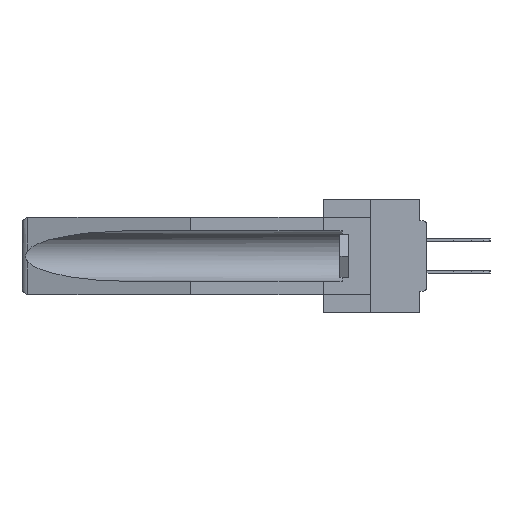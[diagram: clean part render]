
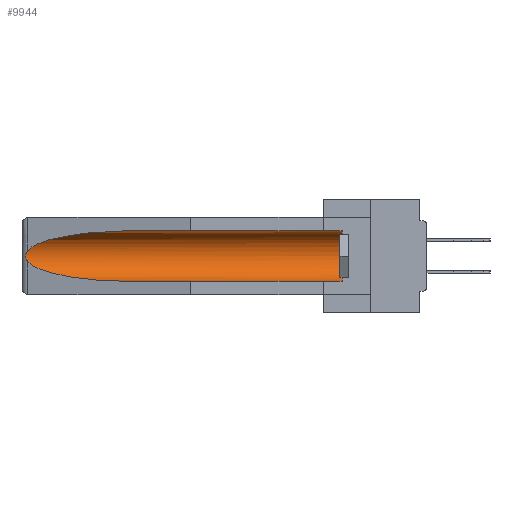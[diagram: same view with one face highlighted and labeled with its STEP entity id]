
A CAD part, left-side view. The second image highlights one B-rep face of the part: STEP entity #9944.
In plain terms, the highlighted cylindrical face has radius 2.857 mm (diameter 5.715 mm), a partial arc.
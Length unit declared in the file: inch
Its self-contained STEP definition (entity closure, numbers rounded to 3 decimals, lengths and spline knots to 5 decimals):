
#399 = CARTESIAN_POINT ( 'NONE',  ( 0.21114, 1.30732, -0.059 ) ) ;
#530 = CARTESIAN_POINT ( 'NONE',  ( 0.155, 1.07973, -0.059 ) ) ;
#977 = DIRECTION ( 'NONE',  ( 0., 1., 0. ) ) ;
#3396 = CARTESIAN_POINT ( 'NONE',  ( 0.25451, 1.48313, -0.09465 ) ) ;
#3493 = CARTESIAN_POINT ( 'NONE',  ( 0.26537, 1.52718, -0.14972 ) ) ;
#3659 = CARTESIAN_POINT ( 'NONE',  ( 0.2673, 1.53269, -0.17917 ) ) ;
#4234 = CARTESIAN_POINT ( 'NONE',  ( 0.155, -0.30754, -0.059 ) ) ;
#4353 = CARTESIAN_POINT ( 'NONE',  ( 0.155, 1.07973, -0.284 ) ) ;
#4997 = VERTEX_POINT ( 'NONE', #4353 ) ;
#5021 = DIRECTION ( 'NONE',  ( 0., -1., 0. ) ) ;
#6024 = CARTESIAN_POINT ( 'NONE',  ( 0.155, 0.126, -0.284 ) ) ;
#6068 = CARTESIAN_POINT ( 'NONE',  ( 0.21114, 1.30732, -0.284 ) ) ;
#7040 = CARTESIAN_POINT ( 'NONE',  ( 0.26654, 1.53092, -0.15636 ) ) ;
#7244 = VERTEX_POINT ( 'NONE', #14159 ) ;
#7848 = CARTESIAN_POINT ( 'NONE',  ( 0.155, 0.126, -0.059 ) ) ;
#7943 = DIRECTION ( 'NONE',  ( 0., 0., 1. ) ) ;
#8507 = AXIS2_PLACEMENT_3D ( 'NONE', #30122, #5021, #26996 ) ;
#8982 = EDGE_CURVE ( 'NONE', #31421, #26354, #31201, .T. ) ;
#9366 = LINE ( 'NONE', #28164, #28283 ) ;
#9666 = ORIENTED_EDGE ( 'NONE', *, *, #23422, .T. ) ;
#9944 = ADVANCED_FACE ( 'NONE', ( #39480 ), #27773, .F. ) ;
#10310 = CARTESIAN_POINT ( 'NONE',  ( 0.2675, 1.53308, -0.17534 ) ) ;
#11092 =( BOUNDED_CURVE ( )  B_SPLINE_CURVE ( 3, ( #27252, #21374, #6068, #27779 ),
 .UNSPECIFIED., .F., .F. ) 
 B_SPLINE_CURVE_WITH_KNOTS ( ( 4, 4 ),
 ( 0.1948, 1.5708 ),
 .UNSPECIFIED. ) 
 CURVE ( )  GEOMETRIC_REPRESENTATION_ITEM ( )  RATIONAL_B_SPLINE_CURVE ( ( 1., 0.848, 0.848, 1. ) ) 
 REPRESENTATION_ITEM ( '' )  );
#14079 = DIRECTION ( 'NONE',  ( 0., 1., 0. ) ) ;
#14159 = CARTESIAN_POINT ( 'NONE',  ( 0.26537, 1.52718, -0.19328 ) ) ;
#14530 = CARTESIAN_POINT ( 'NONE',  ( 0.155, 1.07973, -0.059 ) ) ;
#15015 = EDGE_CURVE ( 'NONE', #18121, #7244, #38730, .T. ) ;
#16290 = CARTESIAN_POINT ( 'NONE',  ( 0.26597, 1.5296, -0.19026 ) ) ;
#16415 = CARTESIAN_POINT ( 'NONE',  ( 0.26537, 1.52718, -0.14972 ) ) ;
#16559 = EDGE_CURVE ( 'NONE', #31421, #4997, #9366, .T. ) ;
#17382 = AXIS2_PLACEMENT_3D ( 'NONE', #26665, #14079, #7943 ) ;
#18121 = VERTEX_POINT ( 'NONE', #3493 ) ;
#18187 = EDGE_LOOP ( 'NONE', ( #9666, #18759, #21582, #34734, #25890, #39552 ) ) ;
#18759 = ORIENTED_EDGE ( 'NONE', *, *, #15015, .T. ) ;
#18803 = DIRECTION ( 'NONE',  ( 0., 1., 0. ) ) ;
#19403 = CARTESIAN_POINT ( 'NONE',  ( 0.26655, 1.53094, -0.18657 ) ) ;
#19683 = VERTEX_POINT ( 'NONE', #14530 ) ;
#21374 = CARTESIAN_POINT ( 'NONE',  ( 0.25451, 1.48313, -0.24835 ) ) ;
#21582 = ORIENTED_EDGE ( 'NONE', *, *, #37620, .T. ) ;
#22199 = CARTESIAN_POINT ( 'NONE',  ( 0.26597, 1.52961, -0.15275 ) ) ;
#23422 = EDGE_CURVE ( 'NONE', #19683, #18121, #24262, .T. ) ;
#24262 =( BOUNDED_CURVE ( )  B_SPLINE_CURVE ( 3, ( #530, #399, #3396, #27813 ),
 .UNSPECIFIED., .F., .F. ) 
 B_SPLINE_CURVE_WITH_KNOTS ( ( 4, 4 ),
 ( 4.71239, 6.08839 ),
 .UNSPECIFIED. ) 
 CURVE ( )  GEOMETRIC_REPRESENTATION_ITEM ( )  RATIONAL_B_SPLINE_CURVE ( ( 1., 0.848, 0.848, 1. ) ) 
 REPRESENTATION_ITEM ( '' )  );
#25419 = VECTOR ( 'NONE', #977, 39.37008 ) ;
#25488 = CARTESIAN_POINT ( 'NONE',  ( 0.2673, 1.5327, -0.16383 ) ) ;
#25885 = CARTESIAN_POINT ( 'NONE',  ( 0.26537, 1.52718, -0.19328 ) ) ;
#25890 = ORIENTED_EDGE ( 'NONE', *, *, #8982, .T. ) ;
#26354 = VERTEX_POINT ( 'NONE', #7848 ) ;
#26665 = CARTESIAN_POINT ( 'NONE',  ( 0.155, -0.30754, -0.1715 ) ) ;
#26996 = DIRECTION ( 'NONE',  ( 0., 0., 1. ) ) ;
#27252 = CARTESIAN_POINT ( 'NONE',  ( 0.26537, 1.52718, -0.19328 ) ) ;
#27773 = CYLINDRICAL_SURFACE ( 'NONE', #17382, 0.1125 ) ;
#27779 = CARTESIAN_POINT ( 'NONE',  ( 0.155, 1.07973, -0.284 ) ) ;
#27813 = CARTESIAN_POINT ( 'NONE',  ( 0.26537, 1.52718, -0.14972 ) ) ;
#28164 = CARTESIAN_POINT ( 'NONE',  ( 0.155, -0.30754, -0.284 ) ) ;
#28283 = VECTOR ( 'NONE', #18803, 39.37008 ) ;
#28877 = CARTESIAN_POINT ( 'NONE',  ( 0.2675, 1.53308, -0.16763 ) ) ;
#30122 = CARTESIAN_POINT ( 'NONE',  ( 0.155, 0.126, -0.1715 ) ) ;
#31201 = CIRCLE ( 'NONE', #8507, 0.1125 ) ;
#31421 = VERTEX_POINT ( 'NONE', #6024 ) ;
#34734 = ORIENTED_EDGE ( 'NONE', *, *, #16559, .F. ) ;
#35441 = EDGE_CURVE ( 'NONE', #26354, #19683, #37108, .T. ) ;
#37108 = LINE ( 'NONE', #4234, #25419 ) ;
#37620 = EDGE_CURVE ( 'NONE', #7244, #4997, #11092, .T. ) ;
#38730 = B_SPLINE_CURVE_WITH_KNOTS ( 'NONE', 3,
 ( #16415, #22199, #7040, #25488, #28877, #10310, #3659, #19403, #16290, #25885 ),
 .UNSPECIFIED., .F., .F.,
 ( 4, 2, 2, 2, 4 ),
 ( 0., 0.00029, 0.00058, 0.00087, 0.00117 ),
 .UNSPECIFIED. ) ;
#39480 = FACE_OUTER_BOUND ( 'NONE', #18187, .T. ) ;
#39552 = ORIENTED_EDGE ( 'NONE', *, *, #35441, .T. ) ;
